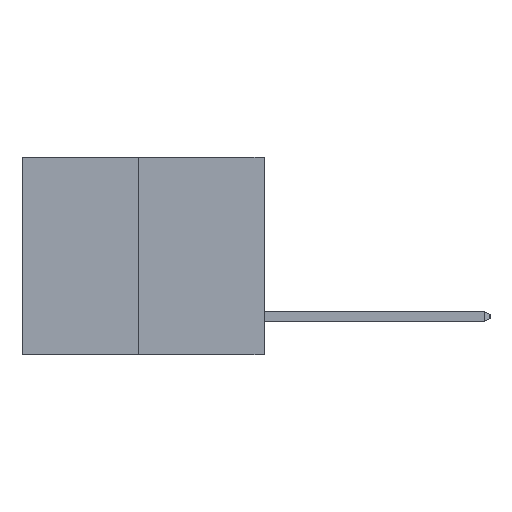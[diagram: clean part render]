
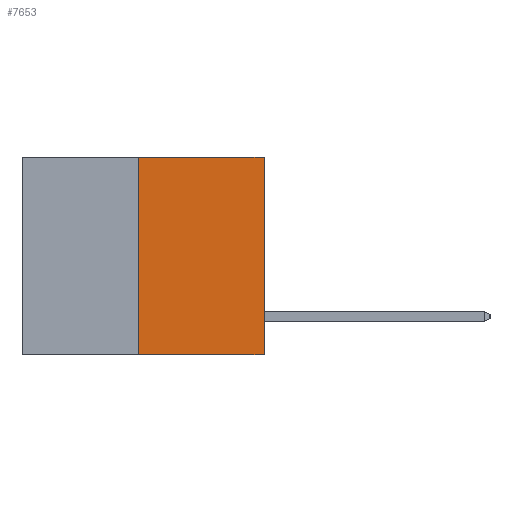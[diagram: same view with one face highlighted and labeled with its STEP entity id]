
A CAD part, left-side view. The second image highlights one B-rep face of the part: STEP entity #7653.
In plain terms, the highlighted planar face has unit normal (-1, 0, 0).
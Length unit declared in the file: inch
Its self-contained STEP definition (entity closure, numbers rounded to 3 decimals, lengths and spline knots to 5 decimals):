
#1563 = AXIS2_PLACEMENT_3D ( 'NONE', #5634, #11851, #26535 ) ;
#1695 = LINE ( 'NONE', #4791, #7178 ) ;
#2368 = ORIENTED_EDGE ( 'NONE', *, *, #23521, .F. ) ;
#2637 = DIRECTION ( 'NONE',  ( 0., -1., 0. ) ) ;
#3288 = CARTESIAN_POINT ( 'NONE',  ( 0., 0.312, -0.49 ) ) ;
#4791 = CARTESIAN_POINT ( 'NONE',  ( 0., 0.6, -0.49 ) ) ;
#4863 = DIRECTION ( 'NONE',  ( 0., 0., 1. ) ) ;
#5634 = CARTESIAN_POINT ( 'NONE',  ( 0., 0.6, 0. ) ) ;
#7178 = VECTOR ( 'NONE', #2637, 39.37008 ) ;
#7653 = ADVANCED_FACE ( 'NONE', ( #16333 ), #9957, .F. ) ;
#7729 = ORIENTED_EDGE ( 'NONE', *, *, #12033, .F. ) ;
#7856 = CARTESIAN_POINT ( 'NONE',  ( 0., 0.312, 0. ) ) ;
#8199 = ORIENTED_EDGE ( 'NONE', *, *, #8564, .T. ) ;
#8564 = EDGE_CURVE ( 'NONE', #11139, #16832, #1695, .T. ) ;
#9846 = ORIENTED_EDGE ( 'NONE', *, *, #21881, .T. ) ;
#9957 = PLANE ( 'NONE',  #1563 ) ;
#10938 = DIRECTION ( 'NONE',  ( 0., 0., 1. ) ) ;
#11139 = VERTEX_POINT ( 'NONE', #3288 ) ;
#11851 = DIRECTION ( 'NONE',  ( 1., 0., 0. ) ) ;
#12033 = EDGE_CURVE ( 'NONE', #25872, #20745, #25845, .T. ) ;
#13268 = CARTESIAN_POINT ( 'NONE',  ( 0., 0., 0. ) ) ;
#13768 = VECTOR ( 'NONE', #4863, 39.37008 ) ;
#15104 = CARTESIAN_POINT ( 'NONE',  ( 0., 0., 0. ) ) ;
#16333 = FACE_OUTER_BOUND ( 'NONE', #17431, .T. ) ;
#16741 = CARTESIAN_POINT ( 'NONE',  ( 0., 0., -0.49 ) ) ;
#16832 = VERTEX_POINT ( 'NONE', #16741 ) ;
#17431 = EDGE_LOOP ( 'NONE', ( #2368, #8199, #9846, #7729 ) ) ;
#18829 = DIRECTION ( 'NONE',  ( 0., -1., 0. ) ) ;
#19456 = CARTESIAN_POINT ( 'NONE',  ( 0., 0.312, -0.49 ) ) ;
#20745 = VERTEX_POINT ( 'NONE', #15104 ) ;
#20787 = VECTOR ( 'NONE', #10938, 39.37008 ) ;
#20894 = LINE ( 'NONE', #13268, #13768 ) ;
#21881 = EDGE_CURVE ( 'NONE', #16832, #20745, #20894, .T. ) ;
#21960 = VECTOR ( 'NONE', #18829, 39.37008 ) ;
#22094 = LINE ( 'NONE', #19456, #20787 ) ;
#23521 = EDGE_CURVE ( 'NONE', #11139, #25872, #22094, .T. ) ;
#24864 = CARTESIAN_POINT ( 'NONE',  ( 0., 0.6, 0. ) ) ;
#25845 = LINE ( 'NONE', #24864, #21960 ) ;
#25872 = VERTEX_POINT ( 'NONE', #7856 ) ;
#26535 = DIRECTION ( 'NONE',  ( 0., 0., -1. ) ) ;
